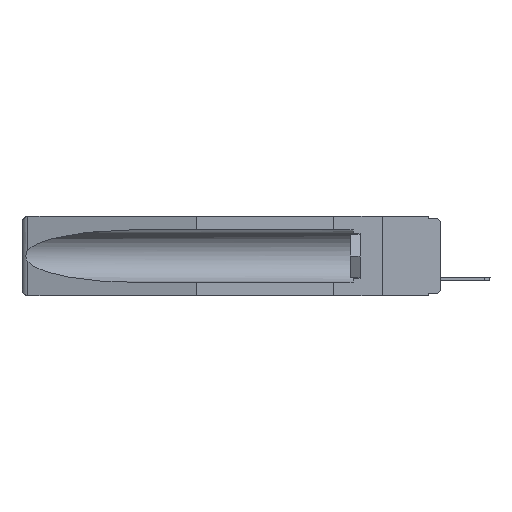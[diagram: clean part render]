
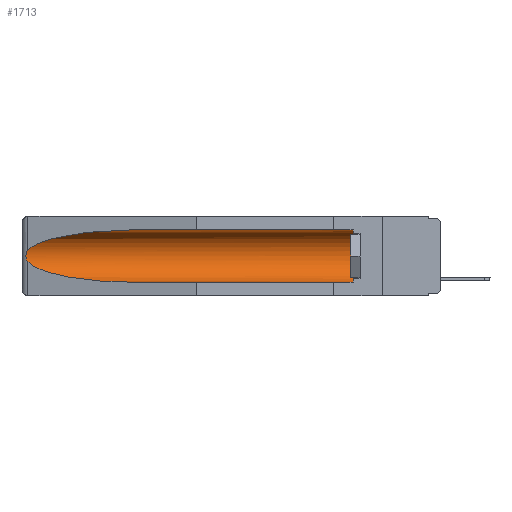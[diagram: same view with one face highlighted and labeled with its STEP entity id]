
A CAD part, left-side view. The second image highlights one B-rep face of the part: STEP entity #1713.
In plain terms, the highlighted cylindrical face has radius 2.857 mm (diameter 5.715 mm), a partial arc.
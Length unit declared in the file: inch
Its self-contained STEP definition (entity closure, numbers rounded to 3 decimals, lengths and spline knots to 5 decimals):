
#427 = EDGE_CURVE ( 'NONE', #14953, #16434, #3765, .T. ) ;
#637 = CARTESIAN_POINT ( 'NONE',  ( 0.21114, 1.30732, -0.284 ) ) ;
#679 = CARTESIAN_POINT ( 'NONE',  ( 0.155, 0.126, -0.059 ) ) ;
#727 = CARTESIAN_POINT ( 'NONE',  ( 0.155, 1.07973, -0.284 ) ) ;
#948 = VECTOR ( 'NONE', #9145, 39.37008 ) ;
#1494 = EDGE_CURVE ( 'NONE', #1763, #8295, #5616, .T. ) ;
#1713 = ADVANCED_FACE ( 'NONE', ( #12857 ), #13906, .F. ) ;
#1758 = CARTESIAN_POINT ( 'NONE',  ( 0.26655, 1.53094, -0.18657 ) ) ;
#1763 = VERTEX_POINT ( 'NONE', #7222 ) ;
#2527 = AXIS2_PLACEMENT_3D ( 'NONE', #7232, #2992, #2903 ) ;
#2893 = CARTESIAN_POINT ( 'NONE',  ( 0.155, -0.30754, -0.1715 ) ) ;
#2903 = DIRECTION ( 'NONE',  ( 0., 0., 1. ) ) ;
#2992 = DIRECTION ( 'NONE',  ( 0., -1., 0. ) ) ;
#3765 = CIRCLE ( 'NONE', #2527, 0.1125 ) ;
#4175 = CARTESIAN_POINT ( 'NONE',  ( 0.155, 0.126, -0.284 ) ) ;
#4491 = CARTESIAN_POINT ( 'NONE',  ( 0.2675, 1.53308, -0.17534 ) ) ;
#4509 = ORIENTED_EDGE ( 'NONE', *, *, #11496, .T. ) ;
#4850 = DIRECTION ( 'NONE',  ( 0., 1., 0. ) ) ;
#5616 =( BOUNDED_CURVE ( )  B_SPLINE_CURVE ( 3, ( #8065, #12003, #637, #727 ),
 .UNSPECIFIED., .F., .F. ) 
 B_SPLINE_CURVE_WITH_KNOTS ( ( 4, 4 ),
 ( 0.1948, 1.5708 ),
 .UNSPECIFIED. ) 
 CURVE ( )  GEOMETRIC_REPRESENTATION_ITEM ( )  RATIONAL_B_SPLINE_CURVE ( ( 1., 0.848, 0.848, 1. ) ) 
 REPRESENTATION_ITEM ( '' )  );
#5673 = CARTESIAN_POINT ( 'NONE',  ( 0.26537, 1.52718, -0.14972 ) ) ;
#5908 = ORIENTED_EDGE ( 'NONE', *, *, #13239, .T. ) ;
#6261 = LINE ( 'NONE', #9269, #15220 ) ;
#6341 = DIRECTION ( 'NONE',  ( 0., 1., 0. ) ) ;
#6654 = EDGE_CURVE ( 'NONE', #14953, #8295, #18000, .T. ) ;
#7222 = CARTESIAN_POINT ( 'NONE',  ( 0.26537, 1.52718, -0.19328 ) ) ;
#7232 = CARTESIAN_POINT ( 'NONE',  ( 0.155, 0.126, -0.1715 ) ) ;
#8065 = CARTESIAN_POINT ( 'NONE',  ( 0.26537, 1.52718, -0.19328 ) ) ;
#8076 = CARTESIAN_POINT ( 'NONE',  ( 0.155, 1.07973, -0.059 ) ) ;
#8295 = VERTEX_POINT ( 'NONE', #11487 ) ;
#8931 = ORIENTED_EDGE ( 'NONE', *, *, #17072, .T. ) ;
#9145 = DIRECTION ( 'NONE',  ( 0., 1., 0. ) ) ;
#9269 = CARTESIAN_POINT ( 'NONE',  ( 0.155, -0.30754, -0.059 ) ) ;
#10136 = CARTESIAN_POINT ( 'NONE',  ( 0.26597, 1.5296, -0.19026 ) ) ;
#10228 = CARTESIAN_POINT ( 'NONE',  ( 0.26537, 1.52718, -0.19328 ) ) ;
#10332 = CARTESIAN_POINT ( 'NONE',  ( 0.21114, 1.30732, -0.059 ) ) ;
#10499 = CARTESIAN_POINT ( 'NONE',  ( 0.26654, 1.53092, -0.15636 ) ) ;
#11051 = EDGE_LOOP ( 'NONE', ( #4509, #8931, #18149, #15719, #15583, #5908 ) ) ;
#11381 = VERTEX_POINT ( 'NONE', #14103 ) ;
#11487 = CARTESIAN_POINT ( 'NONE',  ( 0.155, 1.07973, -0.284 ) ) ;
#11496 = EDGE_CURVE ( 'NONE', #11381, #14882, #16344, .T. ) ;
#11623 = CARTESIAN_POINT ( 'NONE',  ( 0.2675, 1.53308, -0.16763 ) ) ;
#12003 = CARTESIAN_POINT ( 'NONE',  ( 0.25451, 1.48313, -0.24835 ) ) ;
#12857 = FACE_OUTER_BOUND ( 'NONE', #11051, .T. ) ;
#13036 = CARTESIAN_POINT ( 'NONE',  ( 0.26537, 1.52718, -0.14972 ) ) ;
#13239 = EDGE_CURVE ( 'NONE', #16434, #11381, #6261, .T. ) ;
#13397 = AXIS2_PLACEMENT_3D ( 'NONE', #2893, #6341, #17326 ) ;
#13470 = CARTESIAN_POINT ( 'NONE',  ( 0.155, -0.30754, -0.284 ) ) ;
#13906 = CYLINDRICAL_SURFACE ( 'NONE', #13397, 0.1125 ) ;
#14103 = CARTESIAN_POINT ( 'NONE',  ( 0.155, 1.07973, -0.059 ) ) ;
#14295 = CARTESIAN_POINT ( 'NONE',  ( 0.26537, 1.52718, -0.14972 ) ) ;
#14381 = CARTESIAN_POINT ( 'NONE',  ( 0.25451, 1.48313, -0.09465 ) ) ;
#14647 = CARTESIAN_POINT ( 'NONE',  ( 0.26597, 1.52961, -0.15275 ) ) ;
#14882 = VERTEX_POINT ( 'NONE', #5673 ) ;
#14953 = VERTEX_POINT ( 'NONE', #4175 ) ;
#15220 = VECTOR ( 'NONE', #4850, 39.37008 ) ;
#15583 = ORIENTED_EDGE ( 'NONE', *, *, #427, .T. ) ;
#15719 = ORIENTED_EDGE ( 'NONE', *, *, #6654, .F. ) ;
#16344 =( BOUNDED_CURVE ( )  B_SPLINE_CURVE ( 3, ( #8076, #10332, #14381, #14295 ),
 .UNSPECIFIED., .F., .F. ) 
 B_SPLINE_CURVE_WITH_KNOTS ( ( 4, 4 ),
 ( 4.71239, 6.08839 ),
 .UNSPECIFIED. ) 
 CURVE ( )  GEOMETRIC_REPRESENTATION_ITEM ( )  RATIONAL_B_SPLINE_CURVE ( ( 1., 0.848, 0.848, 1. ) ) 
 REPRESENTATION_ITEM ( '' )  );
#16434 = VERTEX_POINT ( 'NONE', #679 ) ;
#17072 = EDGE_CURVE ( 'NONE', #14882, #1763, #17778, .T. ) ;
#17321 = CARTESIAN_POINT ( 'NONE',  ( 0.2673, 1.5327, -0.16383 ) ) ;
#17326 = DIRECTION ( 'NONE',  ( 0., 0., 1. ) ) ;
#17407 = CARTESIAN_POINT ( 'NONE',  ( 0.2673, 1.53269, -0.17917 ) ) ;
#17778 = B_SPLINE_CURVE_WITH_KNOTS ( 'NONE', 3,
 ( #13036, #14647, #10499, #17321, #11623, #4491, #17407, #1758, #10136, #10228 ),
 .UNSPECIFIED., .F., .F.,
 ( 4, 2, 2, 2, 4 ),
 ( 0., 0.00029, 0.00058, 0.00087, 0.00117 ),
 .UNSPECIFIED. ) ;
#18000 = LINE ( 'NONE', #13470, #948 ) ;
#18149 = ORIENTED_EDGE ( 'NONE', *, *, #1494, .T. ) ;
